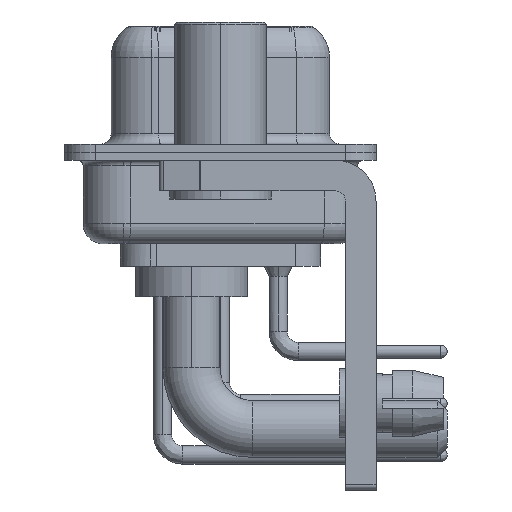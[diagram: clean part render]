
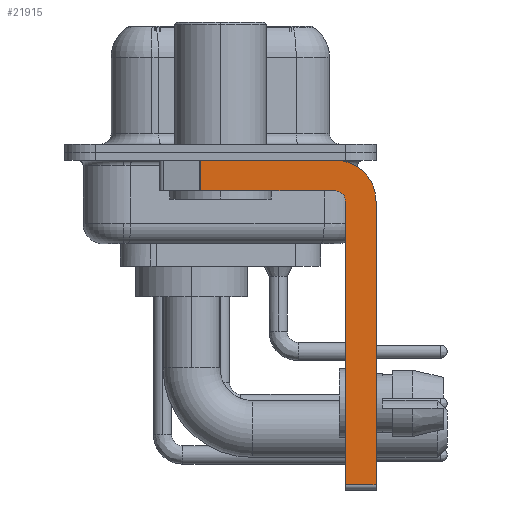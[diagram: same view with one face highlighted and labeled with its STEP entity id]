
A CAD part, left-side view. The second image highlights one B-rep face of the part: STEP entity #21915.
In plain terms, the highlighted planar face has unit normal (-1, 0, 0).
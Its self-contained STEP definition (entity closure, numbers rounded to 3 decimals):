
#476 = DIRECTION ( 'NONE',  ( 0., 1., 0. ) ) ;
#931 = VERTEX_POINT ( 'NONE', #17127 ) ;
#1268 = CARTESIAN_POINT ( 'NONE',  ( -2.9, -5.65, -1.9 ) ) ;
#1947 = DIRECTION ( 'NONE',  ( -1., 0., 0. ) ) ;
#2208 = ORIENTED_EDGE ( 'NONE', *, *, #35871, .F. ) ;
#2406 = EDGE_CURVE ( 'NONE', #29505, #25362, #16169, .T. ) ;
#2576 = CARTESIAN_POINT ( 'NONE',  ( -2.9, 0.978, -0.4 ) ) ;
#2793 = CARTESIAN_POINT ( 'NONE',  ( -2.9, -5.65, -16.35 ) ) ;
#3066 = LINE ( 'NONE', #5642, #3891 ) ;
#3183 = CARTESIAN_POINT ( 'NONE',  ( -2.9, -6.15, -16.6 ) ) ;
#3477 = ORIENTED_EDGE ( 'NONE', *, *, #10127, .F. ) ;
#3891 = VECTOR ( 'NONE', #19335, 1000. ) ;
#5642 = CARTESIAN_POINT ( 'NONE',  ( -2.9, -7.65, -2.4 ) ) ;
#5652 = ORIENTED_EDGE ( 'NONE', *, *, #29781, .F. ) ;
#6214 = VECTOR ( 'NONE', #8956, 1000. ) ;
#7767 = EDGE_CURVE ( 'NONE', #18252, #25362, #30823, .T. ) ;
#7965 = VERTEX_POINT ( 'NONE', #34648 ) ;
#8411 = AXIS2_PLACEMENT_3D ( 'NONE', #10157, #1947, #10527 ) ;
#8686 = LINE ( 'NONE', #3183, #35648 ) ;
#8956 = DIRECTION ( 'NONE',  ( 0., -1., 0. ) ) ;
#9584 = ORIENTED_EDGE ( 'NONE', *, *, #7767, .T. ) ;
#10127 = EDGE_CURVE ( 'NONE', #26708, #931, #3066, .T. ) ;
#10157 = CARTESIAN_POINT ( 'NONE',  ( -2.9, -5.65, -2.4 ) ) ;
#10228 = ORIENTED_EDGE ( 'NONE', *, *, #17665, .F. ) ;
#10527 = DIRECTION ( 'NONE',  ( 0., 0., 1. ) ) ;
#10936 = DIRECTION ( 'NONE',  ( 1., 0., 0. ) ) ;
#11313 = DIRECTION ( 'NONE',  ( 0., 0., -1. ) ) ;
#11438 = CARTESIAN_POINT ( 'NONE',  ( -2.9, 0.978, -1.9 ) ) ;
#11510 = LINE ( 'NONE', #22634, #6214 ) ;
#12975 = ORIENTED_EDGE ( 'NONE', *, *, #35135, .T. ) ;
#13261 = DIRECTION ( 'NONE',  ( 0., 0., -1. ) ) ;
#14230 = AXIS2_PLACEMENT_3D ( 'NONE', #35353, #30399, #13261 ) ;
#14413 = CARTESIAN_POINT ( 'NONE',  ( -2.9, 0.978, -1.9 ) ) ;
#15639 = CARTESIAN_POINT ( 'NONE',  ( -2.9, -6.15, -16.35 ) ) ;
#16169 = LINE ( 'NONE', #17226, #30642 ) ;
#16382 = EDGE_CURVE ( 'NONE', #21142, #29505, #24127, .T. ) ;
#17103 = CARTESIAN_POINT ( 'NONE',  ( -2.9, -5.65, -2.4 ) ) ;
#17127 = CARTESIAN_POINT ( 'NONE',  ( -2.9, -7.65, -16.35 ) ) ;
#17226 = CARTESIAN_POINT ( 'NONE',  ( -2.9, -5.65, -1.9 ) ) ;
#17665 = EDGE_CURVE ( 'NONE', #7965, #26708, #17802, .T. ) ;
#17802 = CIRCLE ( 'NONE', #14230, 2. ) ;
#18060 = ORIENTED_EDGE ( 'NONE', *, *, #16382, .F. ) ;
#18252 = VERTEX_POINT ( 'NONE', #2576 ) ;
#18646 = EDGE_LOOP ( 'NONE', ( #2208, #9584, #30124, #18060, #5652, #12975, #3477, #10228 ) ) ;
#19012 = VECTOR ( 'NONE', #11313, 1000. ) ;
#19335 = DIRECTION ( 'NONE',  ( 0., 0., -1. ) ) ;
#21142 = VERTEX_POINT ( 'NONE', #26293 ) ;
#21915 = ADVANCED_FACE ( 'NONE', ( #30980 ), #22410, .F. ) ;
#22383 = CARTESIAN_POINT ( 'NONE',  ( -2.9, -7.65, -2.4 ) ) ;
#22410 = PLANE ( 'NONE',  #25069 ) ;
#22634 = CARTESIAN_POINT ( 'NONE',  ( -2.9, 3., -0.4 ) ) ;
#24127 = CIRCLE ( 'NONE', #8411, 0.5 ) ;
#25069 = AXIS2_PLACEMENT_3D ( 'NONE', #17103, #10936, #30443 ) ;
#25362 = VERTEX_POINT ( 'NONE', #11438 ) ;
#25446 = DIRECTION ( 'NONE',  ( 0., 0., 1. ) ) ;
#26293 = CARTESIAN_POINT ( 'NONE',  ( -2.9, -6.15, -2.4 ) ) ;
#26533 = VERTEX_POINT ( 'NONE', #15639 ) ;
#26708 = VERTEX_POINT ( 'NONE', #22383 ) ;
#29505 = VERTEX_POINT ( 'NONE', #1268 ) ;
#29781 = EDGE_CURVE ( 'NONE', #26533, #21142, #8686, .T. ) ;
#30124 = ORIENTED_EDGE ( 'NONE', *, *, #2406, .F. ) ;
#30399 = DIRECTION ( 'NONE',  ( 1., 0., 0. ) ) ;
#30443 = DIRECTION ( 'NONE',  ( 0., 0., -1. ) ) ;
#30642 = VECTOR ( 'NONE', #476, 1000. ) ;
#30823 = LINE ( 'NONE', #14413, #19012 ) ;
#30980 = FACE_OUTER_BOUND ( 'NONE', #18646, .T. ) ;
#31837 = VECTOR ( 'NONE', #33103, 1000. ) ;
#33103 = DIRECTION ( 'NONE',  ( 0., -1., 0. ) ) ;
#33642 = LINE ( 'NONE', #2793, #31837 ) ;
#34648 = CARTESIAN_POINT ( 'NONE',  ( -2.9, -5.65, -0.4 ) ) ;
#35135 = EDGE_CURVE ( 'NONE', #26533, #931, #33642, .T. ) ;
#35353 = CARTESIAN_POINT ( 'NONE',  ( -2.9, -5.65, -2.4 ) ) ;
#35648 = VECTOR ( 'NONE', #25446, 1000. ) ;
#35871 = EDGE_CURVE ( 'NONE', #18252, #7965, #11510, .T. ) ;
